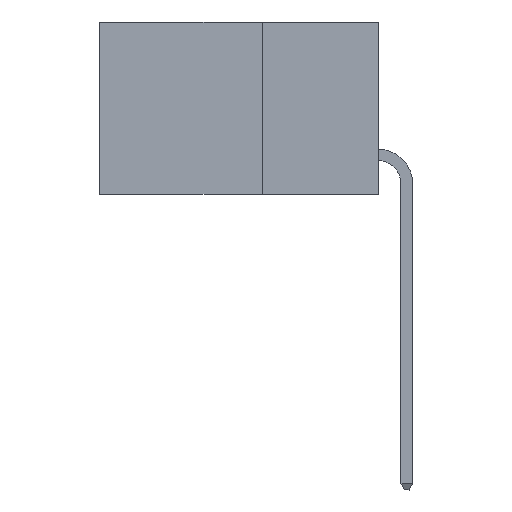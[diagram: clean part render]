
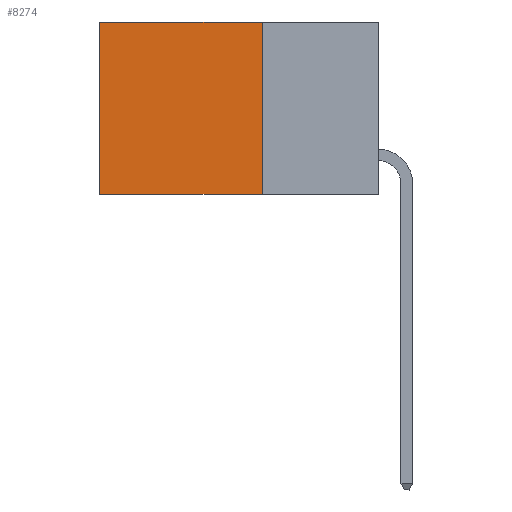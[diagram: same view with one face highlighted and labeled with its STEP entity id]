
A CAD part, left-side view. The second image highlights one B-rep face of the part: STEP entity #8274.
In plain terms, the highlighted planar face has unit normal (-1, 0, 0).
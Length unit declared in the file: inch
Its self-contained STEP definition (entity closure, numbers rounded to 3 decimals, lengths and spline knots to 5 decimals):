
#1105 = ORIENTED_EDGE ( 'NONE', *, *, #7328, .F. ) ;
#2005 = VECTOR ( 'NONE', #6772, 39.37008 ) ;
#2157 = CARTESIAN_POINT ( 'NONE',  ( 0.298, 0.25, 0. ) ) ;
#3008 = EDGE_LOOP ( 'NONE', ( #9694, #1105, #6342, #7528 ) ) ;
#4646 = VERTEX_POINT ( 'NONE', #10486 ) ;
#4697 = AXIS2_PLACEMENT_3D ( 'NONE', #12478, #6466, #13436 ) ;
#4940 = LINE ( 'NONE', #5704, #2005 ) ;
#5374 = LINE ( 'NONE', #11673, #12802 ) ;
#5393 = PLANE ( 'NONE',  #4697 ) ;
#5704 = CARTESIAN_POINT ( 'NONE',  ( 0.298, 0.25, -0.37 ) ) ;
#6342 = ORIENTED_EDGE ( 'NONE', *, *, #7266, .F. ) ;
#6466 = DIRECTION ( 'NONE',  ( 1., 0., 0. ) ) ;
#6725 = CARTESIAN_POINT ( 'NONE',  ( 0.298, 0.25, 0. ) ) ;
#6772 = DIRECTION ( 'NONE',  ( 0., 1., 0. ) ) ;
#7014 = VERTEX_POINT ( 'NONE', #9326 ) ;
#7048 = LINE ( 'NONE', #2157, #9735 ) ;
#7266 = EDGE_CURVE ( 'NONE', #12293, #4646, #10725, .T. ) ;
#7328 = EDGE_CURVE ( 'NONE', #4646, #7014, #4940, .T. ) ;
#7528 = ORIENTED_EDGE ( 'NONE', *, *, #8290, .T. ) ;
#8274 = ADVANCED_FACE ( 'NONE', ( #12968 ), #5393, .F. ) ;
#8290 = EDGE_CURVE ( 'NONE', #12293, #11357, #7048, .T. ) ;
#9207 = EDGE_CURVE ( 'NONE', #11357, #7014, #5374, .T. ) ;
#9326 = CARTESIAN_POINT ( 'NONE',  ( 0.298, 0.6, -0.37 ) ) ;
#9547 = DIRECTION ( 'NONE',  ( 0., 1., 0. ) ) ;
#9694 = ORIENTED_EDGE ( 'NONE', *, *, #9207, .T. ) ;
#9735 = VECTOR ( 'NONE', #9547, 39.37008 ) ;
#10015 = CARTESIAN_POINT ( 'NONE',  ( 0.298, 0.6, 0. ) ) ;
#10486 = CARTESIAN_POINT ( 'NONE',  ( 0.298, 0.25, -0.37 ) ) ;
#10725 = LINE ( 'NONE', #6725, #13286 ) ;
#10767 = DIRECTION ( 'NONE',  ( 0., 0., -1. ) ) ;
#11357 = VERTEX_POINT ( 'NONE', #10015 ) ;
#11627 = DIRECTION ( 'NONE',  ( 0., 0., -1. ) ) ;
#11673 = CARTESIAN_POINT ( 'NONE',  ( 0.298, 0.6, 0. ) ) ;
#12229 = CARTESIAN_POINT ( 'NONE',  ( 0.298, 0.25, 0. ) ) ;
#12293 = VERTEX_POINT ( 'NONE', #12229 ) ;
#12478 = CARTESIAN_POINT ( 'NONE',  ( 0.298, 0.25, 0. ) ) ;
#12802 = VECTOR ( 'NONE', #11627, 39.37008 ) ;
#12968 = FACE_OUTER_BOUND ( 'NONE', #3008, .T. ) ;
#13286 = VECTOR ( 'NONE', #10767, 39.37008 ) ;
#13436 = DIRECTION ( 'NONE',  ( 0., 0., -1. ) ) ;
